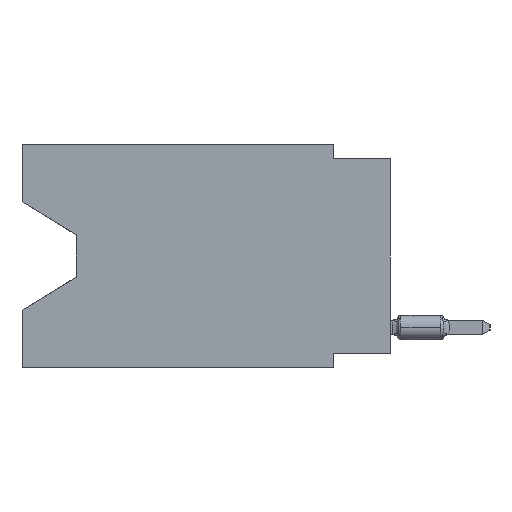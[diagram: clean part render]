
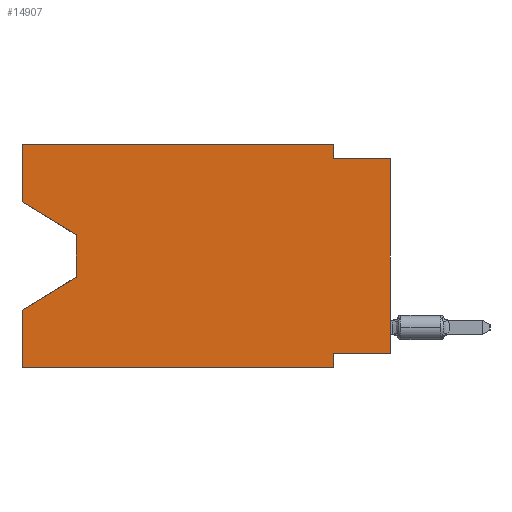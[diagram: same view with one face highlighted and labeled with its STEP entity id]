
A CAD part, left-side view. The second image highlights one B-rep face of the part: STEP entity #14907.
In plain terms, the highlighted planar face has unit normal (-1, 0, 0).
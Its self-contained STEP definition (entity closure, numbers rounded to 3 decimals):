
#205 = VECTOR ( 'NONE', #25083, 1000. ) ;
#404 = EDGE_LOOP ( 'NONE', ( #16821, #19022, #18130, #6923, #7754, #3476, #12144, #20728, #12800, #23111, #4735, #15320 ) ) ;
#445 = CARTESIAN_POINT ( 'NONE',  ( 0., 0., -9.271 ) ) ;
#819 = DIRECTION ( 'NONE',  ( 0., 0., -1. ) ) ;
#952 = VERTEX_POINT ( 'NONE', #19169 ) ;
#1533 = LINE ( 'NONE', #8915, #13234 ) ;
#1539 = EDGE_CURVE ( 'NONE', #16779, #18021, #9610, .T. ) ;
#1784 = CARTESIAN_POINT ( 'NONE',  ( 0., 0., 0. ) ) ;
#1800 = VECTOR ( 'NONE', #17737, 1000. ) ;
#1804 = VERTEX_POINT ( 'NONE', #9287 ) ;
#2272 = CARTESIAN_POINT ( 'NONE',  ( 0., 16.383, -9.906 ) ) ;
#2560 = EDGE_CURVE ( 'NONE', #16886, #10651, #22529, .T. ) ;
#3476 = ORIENTED_EDGE ( 'NONE', *, *, #14069, .F. ) ;
#3903 = EDGE_CURVE ( 'NONE', #20180, #15215, #25811, .T. ) ;
#4003 = LINE ( 'NONE', #1784, #21154 ) ;
#4077 = VECTOR ( 'NONE', #8929, 1000. ) ;
#4635 = CARTESIAN_POINT ( 'NONE',  ( 0., 0., -9.271 ) ) ;
#4735 = ORIENTED_EDGE ( 'NONE', *, *, #16372, .F. ) ;
#4813 = CARTESIAN_POINT ( 'NONE',  ( 0., 16.383, 0. ) ) ;
#4922 = CARTESIAN_POINT ( 'NONE',  ( 0., 2.54, -9.271 ) ) ;
#5173 = VECTOR ( 'NONE', #819, 1000. ) ;
#5277 = DIRECTION ( 'NONE',  ( 0., 0., -1. ) ) ;
#5544 = CARTESIAN_POINT ( 'NONE',  ( 0., 2.54, 0. ) ) ;
#6923 = ORIENTED_EDGE ( 'NONE', *, *, #26152, .F. ) ;
#7104 = VECTOR ( 'NONE', #5277, 1000. ) ;
#7292 = CARTESIAN_POINT ( 'NONE',  ( 0., 16.383, 0. ) ) ;
#7477 = VECTOR ( 'NONE', #15342, 1000. ) ;
#7754 = ORIENTED_EDGE ( 'NONE', *, *, #2560, .T. ) ;
#7884 = VERTEX_POINT ( 'NONE', #23128 ) ;
#8487 = DIRECTION ( 'NONE',  ( 0., 0., -1. ) ) ;
#8915 = CARTESIAN_POINT ( 'NONE',  ( 0., 2.54, -9.906 ) ) ;
#8929 = DIRECTION ( 'NONE',  ( 0., -0.855, -0.519 ) ) ;
#9252 = LINE ( 'NONE', #18261, #14369 ) ;
#9287 = CARTESIAN_POINT ( 'NONE',  ( 0., 0., -0.635 ) ) ;
#9610 = LINE ( 'NONE', #445, #27822 ) ;
#9687 = EDGE_CURVE ( 'NONE', #7884, #952, #21262, .T. ) ;
#9959 = FACE_OUTER_BOUND ( 'NONE', #404, .T. ) ;
#10077 = AXIS2_PLACEMENT_3D ( 'NONE', #7292, #16311, #25343 ) ;
#10202 = CARTESIAN_POINT ( 'NONE',  ( 0., 16.383, 0. ) ) ;
#10651 = VERTEX_POINT ( 'NONE', #14819 ) ;
#12144 = ORIENTED_EDGE ( 'NONE', *, *, #1539, .F. ) ;
#12564 = LINE ( 'NONE', #10202, #27122 ) ;
#12800 = ORIENTED_EDGE ( 'NONE', *, *, #16384, .F. ) ;
#13017 = CARTESIAN_POINT ( 'NONE',  ( 0., 2.54, 0. ) ) ;
#13073 = LINE ( 'NONE', #24173, #4077 ) ;
#13164 = DIRECTION ( 'NONE',  ( 0., 0., 1. ) ) ;
#13234 = VECTOR ( 'NONE', #8487, 1000. ) ;
#13547 = LINE ( 'NONE', #4813, #205 ) ;
#14069 = EDGE_CURVE ( 'NONE', #18021, #10651, #1533, .T. ) ;
#14297 = CARTESIAN_POINT ( 'NONE',  ( 0., 13.97, -4.013 ) ) ;
#14369 = VECTOR ( 'NONE', #27009, 1000. ) ;
#14819 = CARTESIAN_POINT ( 'NONE',  ( 0., 2.54, -9.906 ) ) ;
#14907 = ADVANCED_FACE ( 'NONE', ( #9959 ), #21202, .F. ) ;
#15152 = CARTESIAN_POINT ( 'NONE',  ( 0., 16.383, 0. ) ) ;
#15198 = LINE ( 'NONE', #24223, #7477 ) ;
#15215 = VERTEX_POINT ( 'NONE', #24498 ) ;
#15320 = ORIENTED_EDGE ( 'NONE', *, *, #15735, .F. ) ;
#15342 = DIRECTION ( 'NONE',  ( 0., 0.855, -0.519 ) ) ;
#15722 = DIRECTION ( 'NONE',  ( 0., -1., 0. ) ) ;
#15735 = EDGE_CURVE ( 'NONE', #27743, #23057, #12564, .T. ) ;
#16311 = DIRECTION ( 'NONE',  ( 1., 0., 0. ) ) ;
#16372 = EDGE_CURVE ( 'NONE', #23057, #20180, #13547, .T. ) ;
#16384 = EDGE_CURVE ( 'NONE', #15215, #1804, #9252, .T. ) ;
#16779 = VERTEX_POINT ( 'NONE', #4635 ) ;
#16821 = ORIENTED_EDGE ( 'NONE', *, *, #22987, .T. ) ;
#16886 = VERTEX_POINT ( 'NONE', #25776 ) ;
#17732 = VECTOR ( 'NONE', #15722, 1000. ) ;
#17737 = DIRECTION ( 'NONE',  ( 0., 0., 1. ) ) ;
#17887 = LINE ( 'NONE', #20106, #1800 ) ;
#18021 = VERTEX_POINT ( 'NONE', #4922 ) ;
#18130 = ORIENTED_EDGE ( 'NONE', *, *, #19598, .T. ) ;
#18261 = CARTESIAN_POINT ( 'NONE',  ( 0., 0., -0.635 ) ) ;
#19022 = ORIENTED_EDGE ( 'NONE', *, *, #9687, .T. ) ;
#19169 = CARTESIAN_POINT ( 'NONE',  ( 0., 13.97, -5.893 ) ) ;
#19598 = EDGE_CURVE ( 'NONE', #952, #28392, #15198, .T. ) ;
#20106 = CARTESIAN_POINT ( 'NONE',  ( 0., 16.383, 0. ) ) ;
#20180 = VERTEX_POINT ( 'NONE', #13017 ) ;
#20728 = ORIENTED_EDGE ( 'NONE', *, *, #26287, .T. ) ;
#21154 = VECTOR ( 'NONE', #13164, 1000. ) ;
#21202 = PLANE ( 'NONE',  #10077 ) ;
#21262 = LINE ( 'NONE', #14297, #7104 ) ;
#22529 = LINE ( 'NONE', #2272, #17732 ) ;
#22987 = EDGE_CURVE ( 'NONE', #27743, #7884, #13073, .T. ) ;
#23057 = VERTEX_POINT ( 'NONE', #15152 ) ;
#23111 = ORIENTED_EDGE ( 'NONE', *, *, #3903, .F. ) ;
#23128 = CARTESIAN_POINT ( 'NONE',  ( 0., 13.97, -4.013 ) ) ;
#24173 = CARTESIAN_POINT ( 'NONE',  ( 0., 16.383, -2.546 ) ) ;
#24223 = CARTESIAN_POINT ( 'NONE',  ( 0., 13.97, -5.893 ) ) ;
#24498 = CARTESIAN_POINT ( 'NONE',  ( 0., 2.54, -0.635 ) ) ;
#25083 = DIRECTION ( 'NONE',  ( 0., -1., 0. ) ) ;
#25343 = DIRECTION ( 'NONE',  ( 0., 0., -1. ) ) ;
#25728 = DIRECTION ( 'NONE',  ( 0., 1., 0. ) ) ;
#25776 = CARTESIAN_POINT ( 'NONE',  ( 0., 16.383, -9.906 ) ) ;
#25811 = LINE ( 'NONE', #5544, #5173 ) ;
#25935 = CARTESIAN_POINT ( 'NONE',  ( 0., 16.383, -2.546 ) ) ;
#26152 = EDGE_CURVE ( 'NONE', #16886, #28392, #17887, .T. ) ;
#26287 = EDGE_CURVE ( 'NONE', #16779, #1804, #4003, .T. ) ;
#27009 = DIRECTION ( 'NONE',  ( 0., -1., 0. ) ) ;
#27122 = VECTOR ( 'NONE', #28244, 1000. ) ;
#27743 = VERTEX_POINT ( 'NONE', #25935 ) ;
#27822 = VECTOR ( 'NONE', #25728, 1000. ) ;
#28244 = DIRECTION ( 'NONE',  ( 0., 0., 1. ) ) ;
#28392 = VERTEX_POINT ( 'NONE', #29138 ) ;
#29138 = CARTESIAN_POINT ( 'NONE',  ( 0., 16.383, -7.36 ) ) ;
